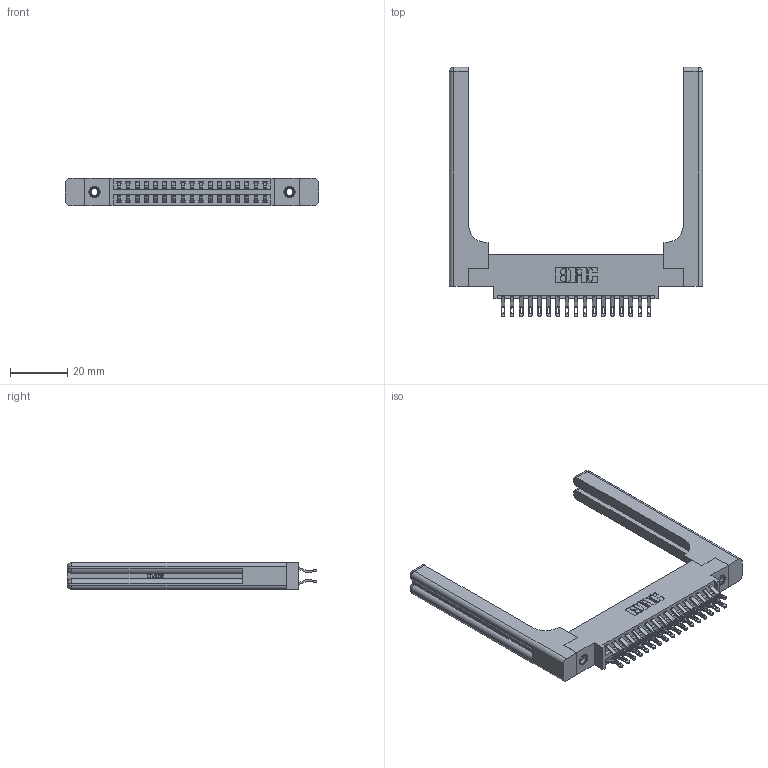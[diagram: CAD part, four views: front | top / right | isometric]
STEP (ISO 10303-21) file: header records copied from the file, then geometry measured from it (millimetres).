
FILE_DESCRIPTION (( 'STEP AP203' ), '1' );
FILE_NAME ('396-034-555-858.STEP', '2019-11-01T20:29:35', ( '' ), ( '' ), 'SwSTEP 2.0', 'SolidWorks 2016', '' );
FILE_SCHEMA (( 'CONFIG_CONTROL_DESIGN' ));
Length unit declared in the file: inch
Products named in the file (5): 346 Part_0.170 Offset - 0.156 Dia-TH; 345-292-001_555 Tail; 345-250-001_345-250-001-102; 346-220-058_345-220-058; 396-034-555-858
Assembly tree (39 placements, depth 2):
  396-034-555-858
    346 Part_0.170 Offset - 0.156 Dia-TH
    345-292-001_555 Tail  x34
    345-250-001_345-250-001-102  x2
    346-220-058_345-220-058  x2
Bounding box: 88.04 x 86.74 x 9.4 mm (x, y, z)
Volume: 15828.7 mm3; surface area: 16567.3 mm2
Topology: 39 solids, 39 shells, 2354 faces, 7229 edges, 4798 vertices
Faces by surface type: plane 1350, cylinder 944, bspline 36, cone 12, sphere 8, torus 4
Entity records: 20100 total; most frequent: CARTESIAN_POINT 4391, ORIENTED_EDGE 3092, DIRECTION 2822, EDGE_CURVE 1546, VECTOR 1234, LINE 1234, VERTEX_POINT 1022, AXIS2_PLACEMENT_3D 794
